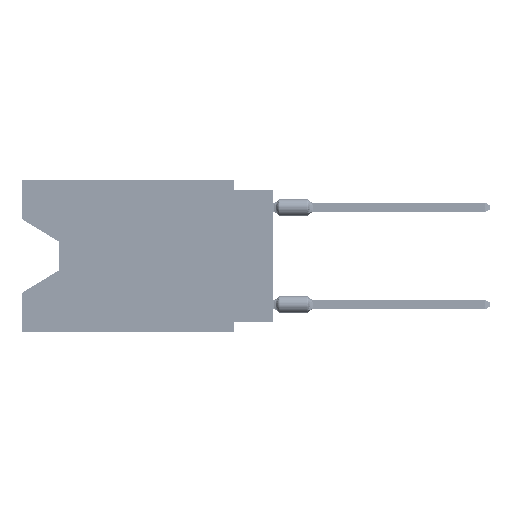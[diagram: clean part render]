
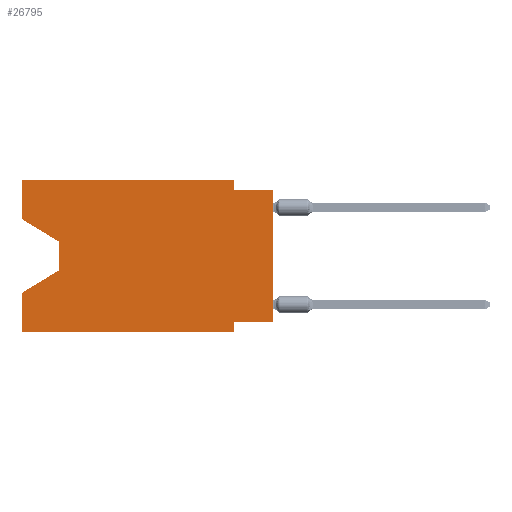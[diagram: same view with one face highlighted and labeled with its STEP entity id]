
A CAD part, left-side view. The second image highlights one B-rep face of the part: STEP entity #26795.
In plain terms, the highlighted planar face has unit normal (-1, 0, 0).
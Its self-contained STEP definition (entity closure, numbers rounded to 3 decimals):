
#815 = VERTEX_POINT ( 'NONE', #65526 ) ;
#979 = EDGE_CURVE ( 'NONE', #8506, #59597, #32396, .T. ) ;
#1221 = CARTESIAN_POINT ( 'NONE',  ( 0., 0., -9.271 ) ) ;
#2036 = CARTESIAN_POINT ( 'NONE',  ( 0., 2.54, 0. ) ) ;
#3739 = EDGE_CURVE ( 'NONE', #64034, #73283, #51816, .T. ) ;
#4550 = CARTESIAN_POINT ( 'NONE',  ( 0., 16.383, 0. ) ) ;
#4784 = LINE ( 'NONE', #35966, #55856 ) ;
#5204 = ORIENTED_EDGE ( 'NONE', *, *, #74194, .T. ) ;
#5869 = VECTOR ( 'NONE', #46689, 1000. ) ;
#6278 = VERTEX_POINT ( 'NONE', #36643 ) ;
#6723 = DIRECTION ( 'NONE',  ( 0., 0., 1. ) ) ;
#8506 = VERTEX_POINT ( 'NONE', #26887 ) ;
#10042 = PLANE ( 'NONE',  #66650 ) ;
#12502 = DIRECTION ( 'NONE',  ( 0., -1., 0. ) ) ;
#13387 = VERTEX_POINT ( 'NONE', #51631 ) ;
#14298 = CARTESIAN_POINT ( 'NONE',  ( 0., 16.383, -9.906 ) ) ;
#15170 = ORIENTED_EDGE ( 'NONE', *, *, #979, .T. ) ;
#15556 = EDGE_CURVE ( 'NONE', #75848, #50110, #43474, .T. ) ;
#15959 = CARTESIAN_POINT ( 'NONE',  ( 0., 16.383, -9.906 ) ) ;
#16955 = DIRECTION ( 'NONE',  ( 0., 0., 1. ) ) ;
#17831 = VECTOR ( 'NONE', #19507, 1000. ) ;
#18415 = LINE ( 'NONE', #1221, #68282 ) ;
#18716 = CARTESIAN_POINT ( 'NONE',  ( 0., 16.383, 0. ) ) ;
#19090 = CARTESIAN_POINT ( 'NONE',  ( 0., 2.54, 0. ) ) ;
#19507 = DIRECTION ( 'NONE',  ( 0., -1., 0. ) ) ;
#20038 = VECTOR ( 'NONE', #35050, 1000. ) ;
#21354 = LINE ( 'NONE', #19090, #49795 ) ;
#22417 = DIRECTION ( 'NONE',  ( 0., 0., -1. ) ) ;
#25153 = ORIENTED_EDGE ( 'NONE', *, *, #41241, .T. ) ;
#25513 = LINE ( 'NONE', #18716, #68287 ) ;
#26305 = CARTESIAN_POINT ( 'NONE',  ( 0., 16.383, -7.36 ) ) ;
#26795 = ADVANCED_FACE ( 'NONE', ( #40403 ), #10042, .F. ) ;
#26887 = CARTESIAN_POINT ( 'NONE',  ( 0., 13.97, -4.013 ) ) ;
#27778 = VECTOR ( 'NONE', #16955, 1000. ) ;
#29510 = LINE ( 'NONE', #40317, #5869 ) ;
#29761 = EDGE_CURVE ( 'NONE', #75848, #70856, #25513, .T. ) ;
#30122 = CARTESIAN_POINT ( 'NONE',  ( 0., 16.383, -2.546 ) ) ;
#32396 = LINE ( 'NONE', #50357, #39090 ) ;
#35050 = DIRECTION ( 'NONE',  ( 0., -1., 0. ) ) ;
#35966 = CARTESIAN_POINT ( 'NONE',  ( 0., 2.54, -9.906 ) ) ;
#35997 = EDGE_CURVE ( 'NONE', #73283, #815, #21354, .T. ) ;
#36643 = CARTESIAN_POINT ( 'NONE',  ( 0., 2.54, -9.271 ) ) ;
#38409 = CARTESIAN_POINT ( 'NONE',  ( 0., 13.97, -5.893 ) ) ;
#39090 = VECTOR ( 'NONE', #62316, 1000. ) ;
#40317 = CARTESIAN_POINT ( 'NONE',  ( 0., 0., 0. ) ) ;
#40403 = FACE_OUTER_BOUND ( 'NONE', #66110, .T. ) ;
#41241 = EDGE_CURVE ( 'NONE', #13387, #51714, #29510, .T. ) ;
#42487 = LINE ( 'NONE', #4550, #27778 ) ;
#42796 = LINE ( 'NONE', #38409, #66710 ) ;
#43474 = LINE ( 'NONE', #14298, #17831 ) ;
#45756 = EDGE_CURVE ( 'NONE', #6278, #50110, #4784, .T. ) ;
#46092 = DIRECTION ( 'NONE',  ( 0., 0., -1. ) ) ;
#46689 = DIRECTION ( 'NONE',  ( 0., 0., 1. ) ) ;
#46910 = DIRECTION ( 'NONE',  ( 0., -0.855, -0.519 ) ) ;
#46947 = ORIENTED_EDGE ( 'NONE', *, *, #35997, .F. ) ;
#49028 = CARTESIAN_POINT ( 'NONE',  ( 0., 2.54, -9.906 ) ) ;
#49090 = CARTESIAN_POINT ( 'NONE',  ( 0., 13.97, -5.893 ) ) ;
#49608 = EDGE_CURVE ( 'NONE', #815, #51714, #60014, .T. ) ;
#49795 = VECTOR ( 'NONE', #46092, 1000. ) ;
#50110 = VERTEX_POINT ( 'NONE', #49028 ) ;
#50357 = CARTESIAN_POINT ( 'NONE',  ( 0., 13.97, -4.013 ) ) ;
#50899 = ORIENTED_EDGE ( 'NONE', *, *, #45756, .F. ) ;
#51470 = ORIENTED_EDGE ( 'NONE', *, *, #77393, .F. ) ;
#51631 = CARTESIAN_POINT ( 'NONE',  ( 0., 0., -9.271 ) ) ;
#51714 = VERTEX_POINT ( 'NONE', #63111 ) ;
#51816 = LINE ( 'NONE', #70514, #20038 ) ;
#52433 = VECTOR ( 'NONE', #12502, 1000. ) ;
#53499 = ORIENTED_EDGE ( 'NONE', *, *, #3739, .F. ) ;
#53905 = EDGE_CURVE ( 'NONE', #58061, #8506, #64844, .T. ) ;
#54714 = ORIENTED_EDGE ( 'NONE', *, *, #15556, .T. ) ;
#55856 = VECTOR ( 'NONE', #71814, 1000. ) ;
#55947 = DIRECTION ( 'NONE',  ( 0., 0.855, -0.519 ) ) ;
#56678 = ORIENTED_EDGE ( 'NONE', *, *, #49608, .F. ) ;
#57742 = ORIENTED_EDGE ( 'NONE', *, *, #29761, .F. ) ;
#58061 = VERTEX_POINT ( 'NONE', #73180 ) ;
#59597 = VERTEX_POINT ( 'NONE', #49090 ) ;
#60014 = LINE ( 'NONE', #73102, #52433 ) ;
#60450 = CARTESIAN_POINT ( 'NONE',  ( 0., 16.383, 0. ) ) ;
#60559 = EDGE_CURVE ( 'NONE', #58061, #64034, #42487, .T. ) ;
#62316 = DIRECTION ( 'NONE',  ( 0., 0., -1. ) ) ;
#63111 = CARTESIAN_POINT ( 'NONE',  ( 0., 0., -0.635 ) ) ;
#64034 = VERTEX_POINT ( 'NONE', #60450 ) ;
#64844 = LINE ( 'NONE', #30122, #72875 ) ;
#65526 = CARTESIAN_POINT ( 'NONE',  ( 0., 2.54, -0.635 ) ) ;
#66110 = EDGE_LOOP ( 'NONE', ( #72722, #15170, #5204, #57742, #54714, #50899, #51470, #25153, #56678, #46947, #53499, #75082 ) ) ;
#66650 = AXIS2_PLACEMENT_3D ( 'NONE', #77042, #77446, #22417 ) ;
#66710 = VECTOR ( 'NONE', #55947, 1000. ) ;
#68282 = VECTOR ( 'NONE', #73039, 1000. ) ;
#68287 = VECTOR ( 'NONE', #6723, 1000. ) ;
#70514 = CARTESIAN_POINT ( 'NONE',  ( 0., 16.383, 0. ) ) ;
#70856 = VERTEX_POINT ( 'NONE', #26305 ) ;
#71814 = DIRECTION ( 'NONE',  ( 0., 0., -1. ) ) ;
#72722 = ORIENTED_EDGE ( 'NONE', *, *, #53905, .T. ) ;
#72875 = VECTOR ( 'NONE', #46910, 1000. ) ;
#73039 = DIRECTION ( 'NONE',  ( 0., 1., 0. ) ) ;
#73102 = CARTESIAN_POINT ( 'NONE',  ( 0., 0., -0.635 ) ) ;
#73180 = CARTESIAN_POINT ( 'NONE',  ( 0., 16.383, -2.546 ) ) ;
#73283 = VERTEX_POINT ( 'NONE', #2036 ) ;
#74194 = EDGE_CURVE ( 'NONE', #59597, #70856, #42796, .T. ) ;
#75082 = ORIENTED_EDGE ( 'NONE', *, *, #60559, .F. ) ;
#75848 = VERTEX_POINT ( 'NONE', #15959 ) ;
#77042 = CARTESIAN_POINT ( 'NONE',  ( 0., 16.383, 0. ) ) ;
#77393 = EDGE_CURVE ( 'NONE', #13387, #6278, #18415, .T. ) ;
#77446 = DIRECTION ( 'NONE',  ( 1., 0., 0. ) ) ;
